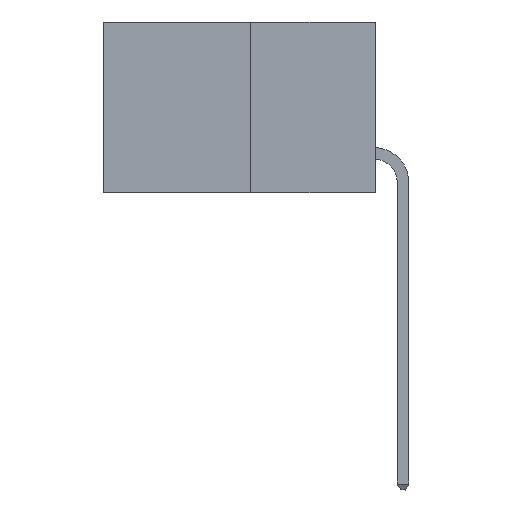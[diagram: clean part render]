
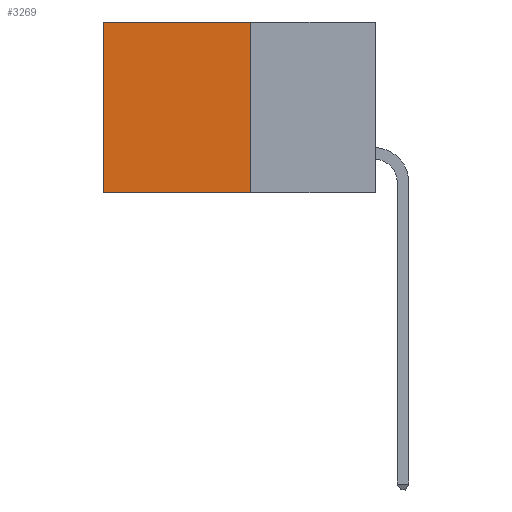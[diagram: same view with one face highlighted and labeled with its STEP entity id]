
A CAD part, left-side view. The second image highlights one B-rep face of the part: STEP entity #3269.
In plain terms, the highlighted planar face has unit normal (-1, 0, 0).
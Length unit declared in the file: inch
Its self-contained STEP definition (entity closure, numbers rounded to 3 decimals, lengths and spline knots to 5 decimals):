
#470 = ORIENTED_EDGE ( 'NONE', *, *, #13653, .T. ) ;
#1896 = CARTESIAN_POINT ( 'NONE',  ( 0.277, 0.59, -0.37 ) ) ;
#1983 = ORIENTED_EDGE ( 'NONE', *, *, #13469, .T. ) ;
#3238 = VECTOR ( 'NONE', #14542, 39.37008 ) ;
#3269 = ADVANCED_FACE ( 'NONE', ( #13026 ), #13768, .F. ) ;
#4276 = CARTESIAN_POINT ( 'NONE',  ( 0.277, 0.27, -0.37 ) ) ;
#4533 = ORIENTED_EDGE ( 'NONE', *, *, #16308, .F. ) ;
#5248 = VECTOR ( 'NONE', #21340, 39.37008 ) ;
#5448 = VERTEX_POINT ( 'NONE', #14501 ) ;
#6642 = CARTESIAN_POINT ( 'NONE',  ( 0.277, 0.59, -0.37 ) ) ;
#6710 = DIRECTION ( 'NONE',  ( 0., 0., -1. ) ) ;
#7351 = DIRECTION ( 'NONE',  ( 0., 0., -1. ) ) ;
#7365 = EDGE_CURVE ( 'NONE', #16594, #5448, #20428, .T. ) ;
#8569 = DIRECTION ( 'NONE',  ( 1., 0., 0. ) ) ;
#10849 = CARTESIAN_POINT ( 'NONE',  ( 0.277, 0.27, -0.37 ) ) ;
#11106 = LINE ( 'NONE', #1896, #16595 ) ;
#11430 = EDGE_LOOP ( 'NONE', ( #1983, #4533, #19575, #470 ) ) ;
#13026 = FACE_OUTER_BOUND ( 'NONE', #11430, .T. ) ;
#13469 = EDGE_CURVE ( 'NONE', #28088, #20889, #11106, .T. ) ;
#13653 = EDGE_CURVE ( 'NONE', #16594, #28088, #23823, .T. ) ;
#13768 = PLANE ( 'NONE',  #21454 ) ;
#14301 = CARTESIAN_POINT ( 'NONE',  ( 0.277, 0.27, -0.37 ) ) ;
#14331 = CARTESIAN_POINT ( 'NONE',  ( 0.277, 0.27, 0. ) ) ;
#14501 = CARTESIAN_POINT ( 'NONE',  ( 0.277, 0.27, -0.37 ) ) ;
#14542 = DIRECTION ( 'NONE',  ( 0., 0., -1. ) ) ;
#15542 = DIRECTION ( 'NONE',  ( 0., 1., 0. ) ) ;
#16121 = LINE ( 'NONE', #10849, #27597 ) ;
#16308 = EDGE_CURVE ( 'NONE', #5448, #20889, #16121, .T. ) ;
#16594 = VERTEX_POINT ( 'NONE', #14331 ) ;
#16595 = VECTOR ( 'NONE', #6710, 39.37008 ) ;
#16697 = CARTESIAN_POINT ( 'NONE',  ( 0.277, 0.27, 0. ) ) ;
#19575 = ORIENTED_EDGE ( 'NONE', *, *, #7365, .F. ) ;
#20428 = LINE ( 'NONE', #14301, #3238 ) ;
#20889 = VERTEX_POINT ( 'NONE', #6642 ) ;
#21340 = DIRECTION ( 'NONE',  ( 0., 1., 0. ) ) ;
#21454 = AXIS2_PLACEMENT_3D ( 'NONE', #4276, #8569, #7351 ) ;
#23823 = LINE ( 'NONE', #16697, #5248 ) ;
#27121 = CARTESIAN_POINT ( 'NONE',  ( 0.277, 0.59, 0. ) ) ;
#27597 = VECTOR ( 'NONE', #15542, 39.37008 ) ;
#28088 = VERTEX_POINT ( 'NONE', #27121 ) ;
